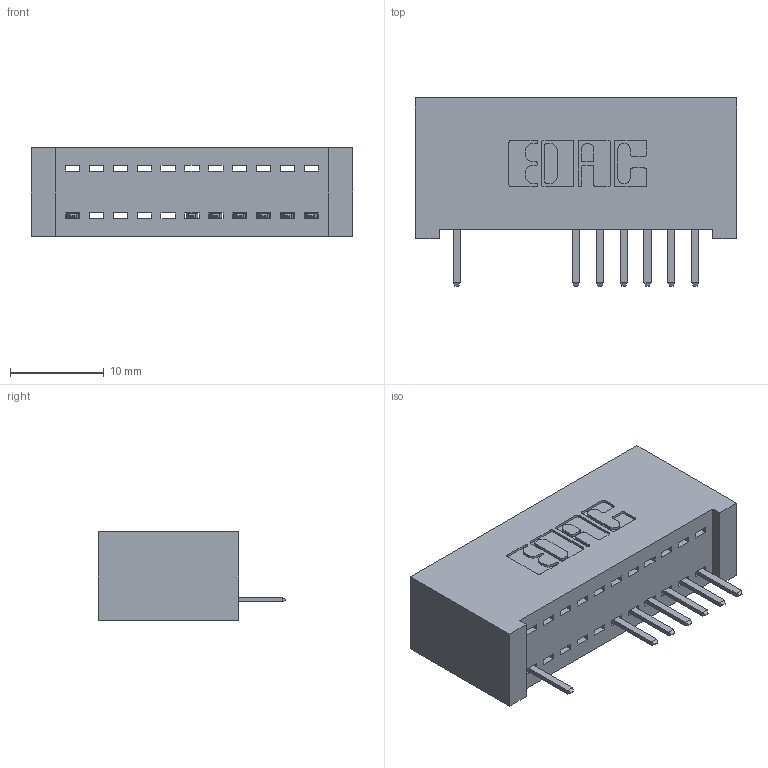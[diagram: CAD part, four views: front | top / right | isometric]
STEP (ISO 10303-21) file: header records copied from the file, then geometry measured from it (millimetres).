
FILE_DESCRIPTION (( 'STEP AP203' ), '1' );
FILE_NAME ('392-011-520-101.STEP', '2018-08-14T21:07:08', ( '' ), ( '' ), 'SwSTEP 2.0', 'SolidWorks 2016', '' );
FILE_SCHEMA (( 'CONFIG_CONTROL_DESIGN' ));
Length unit declared in the file: inch
Products named in the file (3): 345-292-001_345-293-120; 392-011-520-101; 342 Part_Lugless
Assembly tree (8 placements, depth 2):
  392-011-520-101
    342 Part_Lugless
    345-292-001_345-293-120  x7
Bounding box: 34.19 x 20.02 x 9.4 mm (x, y, z)
Volume: 3226.6 mm3; surface area: 4181.1 mm2
Topology: 8 solids, 8 shells, 584 faces, 1731 edges, 1134 vertices
Faces by surface type: plane 418, cylinder 166
Entity records: 10311 total; most frequent: CARTESIAN_POINT 1819, ORIENTED_EDGE 1758, DIRECTION 1573, EDGE_CURVE 879, LINE 755, VECTOR 755, VERTEX_POINT 582, AXIS2_PLACEMENT_3D 409
